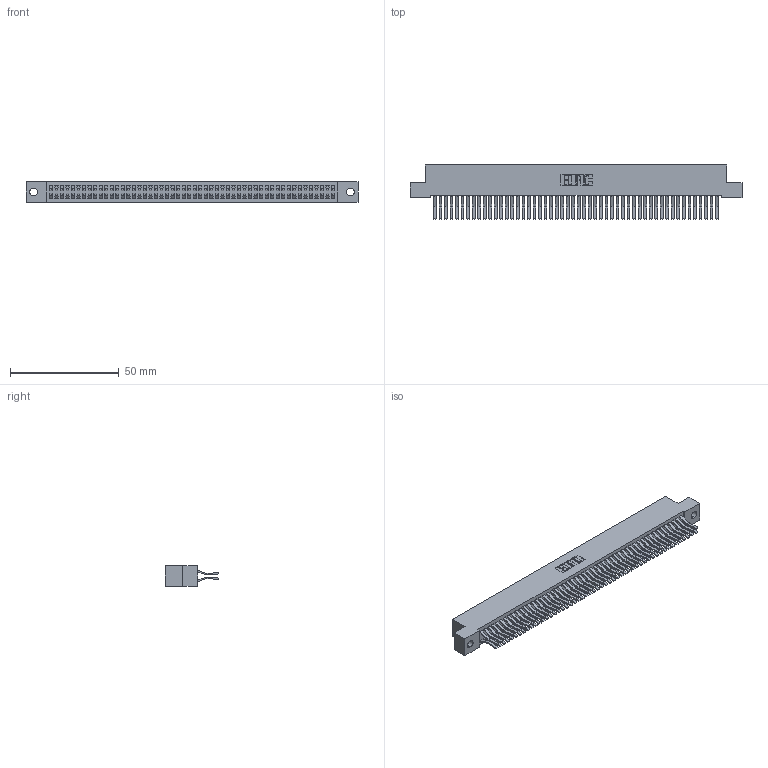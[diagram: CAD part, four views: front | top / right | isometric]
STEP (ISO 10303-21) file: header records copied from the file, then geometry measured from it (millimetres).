
FILE_DESCRIPTION (( 'STEP AP203' ), '1' );
FILE_NAME ('392-104-560-202.STEP', '2019-10-09T22:17:21', ( '' ), ( '' ), 'SwSTEP 2.0', 'SolidWorks 2016', '' );
FILE_SCHEMA (( 'CONFIG_CONTROL_DESIGN' ));
Length unit declared in the file: inch
Products named in the file (3): 342 Part_.128 Slot; 345-292-001_560 Tail; 392-104-560-202
Assembly tree (105 placements, depth 2):
  392-104-560-202
    342 Part_.128 Slot
    345-292-001_560 Tail  x104
Bounding box: 152.4 x 24.78 x 9.4 mm (x, y, z)
Volume: 14371.1 mm3; surface area: 25035.7 mm2
Topology: 105 solids, 105 shells, 5730 faces, 17055 edges, 11230 vertices
Faces by surface type: plane 3814, cylinder 1916
Entity records: 32251 total; most frequent: CARTESIAN_POINT 5334, ORIENTED_EDGE 5270, DIRECTION 4543, EDGE_CURVE 2635, LINE 2503, VECTOR 2503, VERTEX_POINT 1754, AXIS2_PLACEMENT_3D 1020
